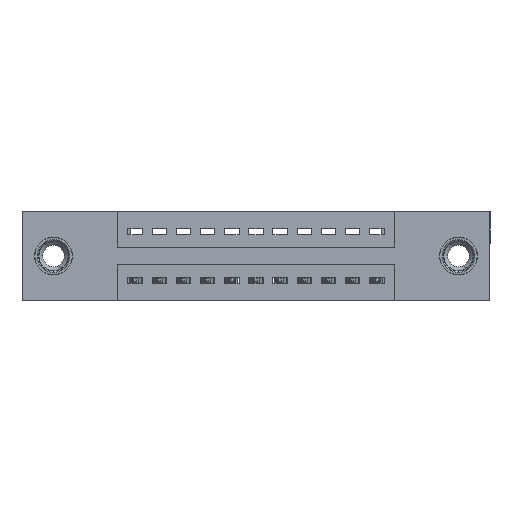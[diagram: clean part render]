
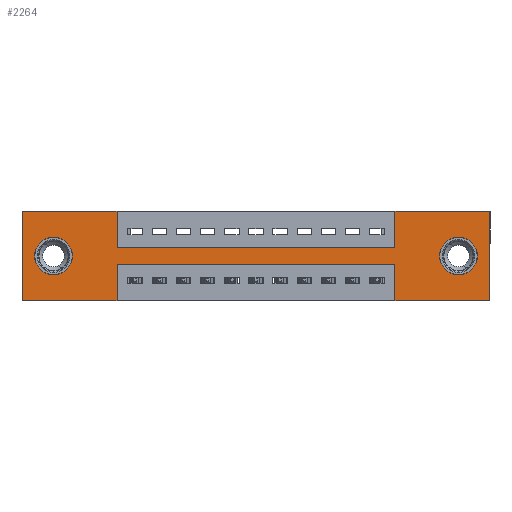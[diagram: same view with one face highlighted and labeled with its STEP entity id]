
A CAD part, front view. The second image highlights one B-rep face of the part: STEP entity #2264.
In plain terms, the highlighted planar face has unit normal (0, -1, 0).
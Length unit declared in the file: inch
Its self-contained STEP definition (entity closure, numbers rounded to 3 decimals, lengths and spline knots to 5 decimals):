
#459 = ORIENTED_EDGE ( 'NONE', *, *, #8148, .F. ) ;
#608 = DIRECTION ( 'NONE',  ( 0., 0., -1. ) ) ;
#995 = DIRECTION ( 'NONE',  ( 0., 1., 0. ) ) ;
#1065 = FACE_BOUND ( 'NONE', #12104, .T. ) ;
#1081 = CARTESIAN_POINT ( 'NONE',  ( 1.5425, 0., 0. ) ) ;
#1122 = VERTEX_POINT ( 'NONE', #1923 ) ;
#1190 = AXIS2_PLACEMENT_3D ( 'NONE', #6886, #995, #7826 ) ;
#1202 = EDGE_CURVE ( 'NONE', #2108, #3866, #8728, .T. ) ;
#1221 = LINE ( 'NONE', #4996, #11687 ) ;
#1358 = CARTESIAN_POINT ( 'NONE',  ( 1.935, 0., 0. ) ) ;
#1386 = EDGE_LOOP ( 'NONE', ( #7897, #9407, #14256, #14302, #3485, #3700, #459, #6219, #4062, #13959, #3400, #9491 ) ) ;
#1392 = DIRECTION ( 'NONE',  ( 0., 0., 1. ) ) ;
#1534 = VECTOR ( 'NONE', #8119, 39.37008 ) ;
#1572 = CARTESIAN_POINT ( 'NONE',  ( 0.3925, 0., 0. ) ) ;
#1588 = VECTOR ( 'NONE', #8599, 39.37008 ) ;
#1923 = CARTESIAN_POINT ( 'NONE',  ( 1.5425, 0., -0.37 ) ) ;
#1984 = CARTESIAN_POINT ( 'NONE',  ( 0., 0., 0. ) ) ;
#2108 = VERTEX_POINT ( 'NONE', #2655 ) ;
#2150 = DIRECTION ( 'NONE',  ( 0., 0., 1. ) ) ;
#2196 = ORIENTED_EDGE ( 'NONE', *, *, #1202, .T. ) ;
#2228 = CARTESIAN_POINT ( 'NONE',  ( 0.13, 0., -0.185 ) ) ;
#2263 = AXIS2_PLACEMENT_3D ( 'NONE', #2228, #14632, #1392 ) ;
#2264 = ADVANCED_FACE ( 'NONE', ( #9042, #1065, #8696 ), #3277, .T. ) ;
#2285 = DIRECTION ( 'NONE',  ( 0., 0., 1. ) ) ;
#2408 = CARTESIAN_POINT ( 'NONE',  ( 0.3925, 0., -0.37 ) ) ;
#2500 = VECTOR ( 'NONE', #3957, 39.37008 ) ;
#2655 = CARTESIAN_POINT ( 'NONE',  ( 0.13, 0., -0.263 ) ) ;
#2859 = DIRECTION ( 'NONE',  ( 0., 1., 0. ) ) ;
#2910 = EDGE_CURVE ( 'NONE', #11130, #4395, #6197, .T. ) ;
#2939 = AXIS2_PLACEMENT_3D ( 'NONE', #5041, #4011, #608 ) ;
#3014 = DIRECTION ( 'NONE',  ( 0., 0., -1. ) ) ;
#3172 = VECTOR ( 'NONE', #12620, 39.37008 ) ;
#3197 = CARTESIAN_POINT ( 'NONE',  ( 0.3925, 0., 0. ) ) ;
#3201 = CIRCLE ( 'NONE', #2263, 0.078 ) ;
#3210 = CARTESIAN_POINT ( 'NONE',  ( 1.935, 0., 0. ) ) ;
#3277 = PLANE ( 'NONE',  #4167 ) ;
#3330 = VERTEX_POINT ( 'NONE', #9154 ) ;
#3400 = ORIENTED_EDGE ( 'NONE', *, *, #10788, .F. ) ;
#3485 = ORIENTED_EDGE ( 'NONE', *, *, #6930, .F. ) ;
#3548 = CARTESIAN_POINT ( 'NONE',  ( 0.3925, 0., -0.37 ) ) ;
#3700 = ORIENTED_EDGE ( 'NONE', *, *, #11225, .F. ) ;
#3866 = VERTEX_POINT ( 'NONE', #12990 ) ;
#3957 = DIRECTION ( 'NONE',  ( -1., 0., 0. ) ) ;
#4011 = DIRECTION ( 'NONE',  ( 0., 1., 0. ) ) ;
#4062 = ORIENTED_EDGE ( 'NONE', *, *, #10525, .F. ) ;
#4149 = EDGE_CURVE ( 'NONE', #3330, #5667, #13747, .T. ) ;
#4167 = AXIS2_PLACEMENT_3D ( 'NONE', #5628, #11323, #6766 ) ;
#4395 = VERTEX_POINT ( 'NONE', #5586 ) ;
#4457 = LINE ( 'NONE', #13360, #2500 ) ;
#4718 = CARTESIAN_POINT ( 'NONE',  ( 0.3925, 0., -0.15 ) ) ;
#4858 = VERTEX_POINT ( 'NONE', #8615 ) ;
#4996 = CARTESIAN_POINT ( 'NONE',  ( 0., 0., 0. ) ) ;
#5041 = CARTESIAN_POINT ( 'NONE',  ( 1.805, 0., -0.185 ) ) ;
#5066 = CARTESIAN_POINT ( 'NONE',  ( 0., 0., -0.37 ) ) ;
#5586 = CARTESIAN_POINT ( 'NONE',  ( 0., 0., -0.37 ) ) ;
#5628 = CARTESIAN_POINT ( 'NONE',  ( 0., 0., -0.37 ) ) ;
#5667 = VERTEX_POINT ( 'NONE', #8228 ) ;
#5831 = VERTEX_POINT ( 'NONE', #11337 ) ;
#5978 = CARTESIAN_POINT ( 'NONE',  ( 0., 0., 0. ) ) ;
#6086 = ORIENTED_EDGE ( 'NONE', *, *, #9454, .T. ) ;
#6197 = LINE ( 'NONE', #5066, #12910 ) ;
#6219 = ORIENTED_EDGE ( 'NONE', *, *, #14588, .F. ) ;
#6766 = DIRECTION ( 'NONE',  ( 0., 0., -1. ) ) ;
#6818 = LINE ( 'NONE', #1358, #11946 ) ;
#6886 = CARTESIAN_POINT ( 'NONE',  ( 0.13, 0., -0.185 ) ) ;
#6930 = EDGE_CURVE ( 'NONE', #10373, #9198, #6818, .T. ) ;
#7111 = CARTESIAN_POINT ( 'NONE',  ( 0., 0., 0. ) ) ;
#7184 = AXIS2_PLACEMENT_3D ( 'NONE', #7371, #2859, #9656 ) ;
#7286 = ORIENTED_EDGE ( 'NONE', *, *, #4149, .T. ) ;
#7367 = EDGE_LOOP ( 'NONE', ( #7286, #6086 ) ) ;
#7371 = CARTESIAN_POINT ( 'NONE',  ( 1.805, 0., -0.185 ) ) ;
#7512 = ORIENTED_EDGE ( 'NONE', *, *, #10449, .T. ) ;
#7597 = VERTEX_POINT ( 'NONE', #11125 ) ;
#7826 = DIRECTION ( 'NONE',  ( 0., 0., 1. ) ) ;
#7897 = ORIENTED_EDGE ( 'NONE', *, *, #11114, .F. ) ;
#8119 = DIRECTION ( 'NONE',  ( 1., 0., 0. ) ) ;
#8148 = EDGE_CURVE ( 'NONE', #7597, #4858, #14528, .T. ) ;
#8228 = CARTESIAN_POINT ( 'NONE',  ( 1.805, 0., -0.263 ) ) ;
#8317 = VECTOR ( 'NONE', #9900, 39.37008 ) ;
#8599 = DIRECTION ( 'NONE',  ( 1., 0., 0. ) ) ;
#8615 = CARTESIAN_POINT ( 'NONE',  ( 1.5425, 0., 0. ) ) ;
#8668 = LINE ( 'NONE', #5978, #1588 ) ;
#8696 = FACE_OUTER_BOUND ( 'NONE', #1386, .T. ) ;
#8728 = CIRCLE ( 'NONE', #1190, 0.078 ) ;
#9042 = FACE_BOUND ( 'NONE', #7367, .T. ) ;
#9046 = CARTESIAN_POINT ( 'NONE',  ( 1.5425, 0., -0.37 ) ) ;
#9112 = VERTEX_POINT ( 'NONE', #7111 ) ;
#9154 = CARTESIAN_POINT ( 'NONE',  ( 1.805, 0., -0.107 ) ) ;
#9177 = LINE ( 'NONE', #9046, #12886 ) ;
#9198 = VERTEX_POINT ( 'NONE', #10459 ) ;
#9370 = CARTESIAN_POINT ( 'NONE',  ( 0.3925, 0., -0.22 ) ) ;
#9407 = ORIENTED_EDGE ( 'NONE', *, *, #13465, .F. ) ;
#9454 = EDGE_CURVE ( 'NONE', #5667, #3330, #13105, .T. ) ;
#9491 = ORIENTED_EDGE ( 'NONE', *, *, #2910, .F. ) ;
#9610 = VECTOR ( 'NONE', #2150, 39.37008 ) ;
#9656 = DIRECTION ( 'NONE',  ( 0., 0., -1. ) ) ;
#9900 = DIRECTION ( 'NONE',  ( 1., 0., 0. ) ) ;
#9998 = CARTESIAN_POINT ( 'NONE',  ( 0.3925, 0., -0.22 ) ) ;
#10069 = LINE ( 'NONE', #9370, #3172 ) ;
#10078 = VECTOR ( 'NONE', #3014, 39.37008 ) ;
#10102 = CARTESIAN_POINT ( 'NONE',  ( 1.5425, 0., -0.22 ) ) ;
#10287 = VERTEX_POINT ( 'NONE', #10102 ) ;
#10373 = VERTEX_POINT ( 'NONE', #3210 ) ;
#10449 = EDGE_CURVE ( 'NONE', #3866, #2108, #3201, .T. ) ;
#10459 = CARTESIAN_POINT ( 'NONE',  ( 1.935, 0., -0.37 ) ) ;
#10525 = EDGE_CURVE ( 'NONE', #11089, #5831, #13616, .T. ) ;
#10618 = EDGE_CURVE ( 'NONE', #9112, #11089, #8668, .T. ) ;
#10661 = VECTOR ( 'NONE', #11774, 39.37008 ) ;
#10788 = EDGE_CURVE ( 'NONE', #4395, #9112, #1221, .T. ) ;
#11089 = VERTEX_POINT ( 'NONE', #3197 ) ;
#11114 = EDGE_CURVE ( 'NONE', #11227, #11130, #12020, .T. ) ;
#11125 = CARTESIAN_POINT ( 'NONE',  ( 1.5425, 0., -0.15 ) ) ;
#11130 = VERTEX_POINT ( 'NONE', #2408 ) ;
#11225 = EDGE_CURVE ( 'NONE', #4858, #10373, #11315, .T. ) ;
#11227 = VERTEX_POINT ( 'NONE', #9998 ) ;
#11264 = EDGE_CURVE ( 'NONE', #1122, #10287, #9177, .T. ) ;
#11315 = LINE ( 'NONE', #1984, #8317 ) ;
#11323 = DIRECTION ( 'NONE',  ( 0., -1., 0. ) ) ;
#11337 = CARTESIAN_POINT ( 'NONE',  ( 0.3925, 0., -0.15 ) ) ;
#11633 = LINE ( 'NONE', #4718, #1534 ) ;
#11687 = VECTOR ( 'NONE', #12884, 39.37008 ) ;
#11698 = EDGE_CURVE ( 'NONE', #9198, #1122, #4457, .T. ) ;
#11719 = DIRECTION ( 'NONE',  ( 0., 0., -1. ) ) ;
#11774 = DIRECTION ( 'NONE',  ( 0., 0., -1. ) ) ;
#11946 = VECTOR ( 'NONE', #11719, 39.37008 ) ;
#12020 = LINE ( 'NONE', #3548, #10078 ) ;
#12104 = EDGE_LOOP ( 'NONE', ( #7512, #2196 ) ) ;
#12620 = DIRECTION ( 'NONE',  ( -1., 0., 0. ) ) ;
#12884 = DIRECTION ( 'NONE',  ( 0., 0., 1. ) ) ;
#12886 = VECTOR ( 'NONE', #2285, 39.37008 ) ;
#12903 = DIRECTION ( 'NONE',  ( -1., 0., 0. ) ) ;
#12910 = VECTOR ( 'NONE', #12903, 39.37008 ) ;
#12990 = CARTESIAN_POINT ( 'NONE',  ( 0.13, 0., -0.107 ) ) ;
#13105 = CIRCLE ( 'NONE', #2939, 0.078 ) ;
#13360 = CARTESIAN_POINT ( 'NONE',  ( 0., 0., -0.37 ) ) ;
#13465 = EDGE_CURVE ( 'NONE', #10287, #11227, #10069, .T. ) ;
#13616 = LINE ( 'NONE', #1572, #10661 ) ;
#13747 = CIRCLE ( 'NONE', #7184, 0.078 ) ;
#13959 = ORIENTED_EDGE ( 'NONE', *, *, #10618, .F. ) ;
#14256 = ORIENTED_EDGE ( 'NONE', *, *, #11264, .F. ) ;
#14302 = ORIENTED_EDGE ( 'NONE', *, *, #11698, .F. ) ;
#14528 = LINE ( 'NONE', #1081, #9610 ) ;
#14588 = EDGE_CURVE ( 'NONE', #5831, #7597, #11633, .T. ) ;
#14632 = DIRECTION ( 'NONE',  ( 0., 1., 0. ) ) ;
